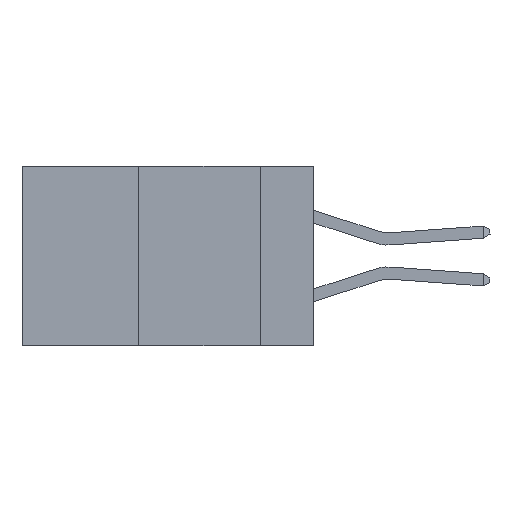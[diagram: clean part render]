
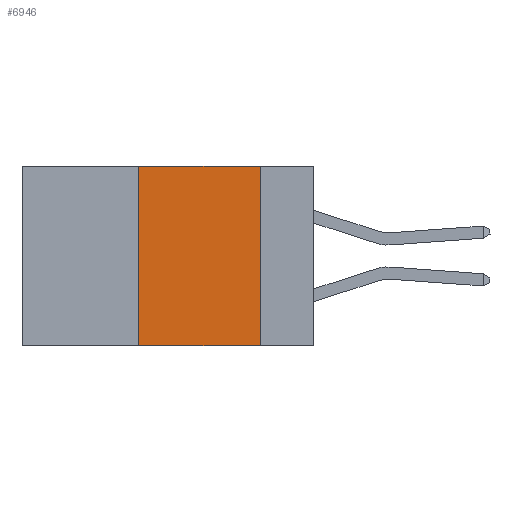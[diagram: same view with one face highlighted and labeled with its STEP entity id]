
A CAD part, left-side view. The second image highlights one B-rep face of the part: STEP entity #6946.
In plain terms, the highlighted planar face has unit normal (-1, 0, 0).
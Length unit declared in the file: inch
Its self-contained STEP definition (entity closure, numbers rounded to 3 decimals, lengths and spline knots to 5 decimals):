
#55 = CARTESIAN_POINT ( 'NONE',  ( 0., 0.6, -0.37 ) ) ;
#143 = LINE ( 'NONE', #55, #14004 ) ;
#188 = DIRECTION ( 'NONE',  ( 0., -1., 0. ) ) ;
#236 = CARTESIAN_POINT ( 'NONE',  ( 0., 0.36, 0. ) ) ;
#442 = CARTESIAN_POINT ( 'NONE',  ( 0., 0.11, 0. ) ) ;
#1081 = VECTOR ( 'NONE', #8083, 39.37008 ) ;
#1465 = CARTESIAN_POINT ( 'NONE',  ( 0., 0.36, -0.37 ) ) ;
#1773 = EDGE_CURVE ( 'NONE', #5544, #12195, #143, .T. ) ;
#2221 = ORIENTED_EDGE ( 'NONE', *, *, #15675, .F. ) ;
#2403 = PLANE ( 'NONE',  #3873 ) ;
#2844 = EDGE_CURVE ( 'NONE', #7611, #12195, #12221, .T. ) ;
#3873 = AXIS2_PLACEMENT_3D ( 'NONE', #6528, #5218, #10559 ) ;
#4252 = CARTESIAN_POINT ( 'NONE',  ( 0., 0.11, -0.37 ) ) ;
#4440 = VECTOR ( 'NONE', #188, 39.37008 ) ;
#4986 = ORIENTED_EDGE ( 'NONE', *, *, #1773, .T. ) ;
#5090 = VERTEX_POINT ( 'NONE', #13583 ) ;
#5218 = DIRECTION ( 'NONE',  ( 1., 0., 0. ) ) ;
#5516 = CARTESIAN_POINT ( 'NONE',  ( 0., 0.11, 0. ) ) ;
#5544 = VERTEX_POINT ( 'NONE', #1465 ) ;
#6083 = ORIENTED_EDGE ( 'NONE', *, *, #16546, .F. ) ;
#6528 = CARTESIAN_POINT ( 'NONE',  ( 0., 0.6, 0. ) ) ;
#6946 = ADVANCED_FACE ( 'NONE', ( #17315 ), #2403, .F. ) ;
#7611 = VERTEX_POINT ( 'NONE', #5516 ) ;
#8083 = DIRECTION ( 'NONE',  ( 0., 0., 1. ) ) ;
#8767 = VECTOR ( 'NONE', #16258, 39.37008 ) ;
#9278 = CARTESIAN_POINT ( 'NONE',  ( 0., 0.6, 0. ) ) ;
#10559 = DIRECTION ( 'NONE',  ( 0., 0., -1. ) ) ;
#10646 = EDGE_LOOP ( 'NONE', ( #15968, #6083, #2221, #4986 ) ) ;
#10957 = DIRECTION ( 'NONE',  ( 0., -1., 0. ) ) ;
#12195 = VERTEX_POINT ( 'NONE', #4252 ) ;
#12221 = LINE ( 'NONE', #442, #8767 ) ;
#13337 = LINE ( 'NONE', #236, #1081 ) ;
#13467 = LINE ( 'NONE', #9278, #4440 ) ;
#13583 = CARTESIAN_POINT ( 'NONE',  ( 0., 0.36, 0. ) ) ;
#14004 = VECTOR ( 'NONE', #10957, 39.37008 ) ;
#15675 = EDGE_CURVE ( 'NONE', #5544, #5090, #13337, .T. ) ;
#15968 = ORIENTED_EDGE ( 'NONE', *, *, #2844, .F. ) ;
#16258 = DIRECTION ( 'NONE',  ( 0., 0., -1. ) ) ;
#16546 = EDGE_CURVE ( 'NONE', #5090, #7611, #13467, .T. ) ;
#17315 = FACE_OUTER_BOUND ( 'NONE', #10646, .T. ) ;
